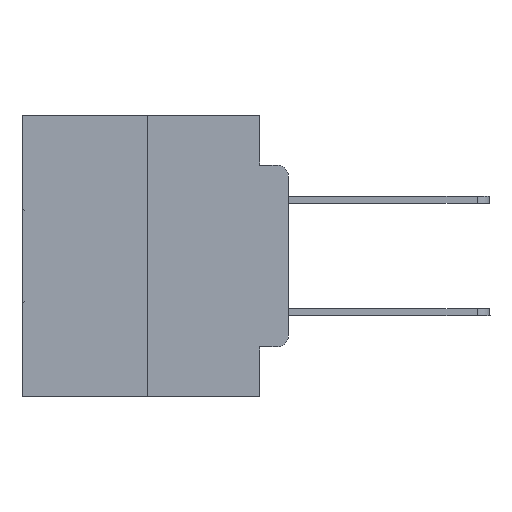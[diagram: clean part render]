
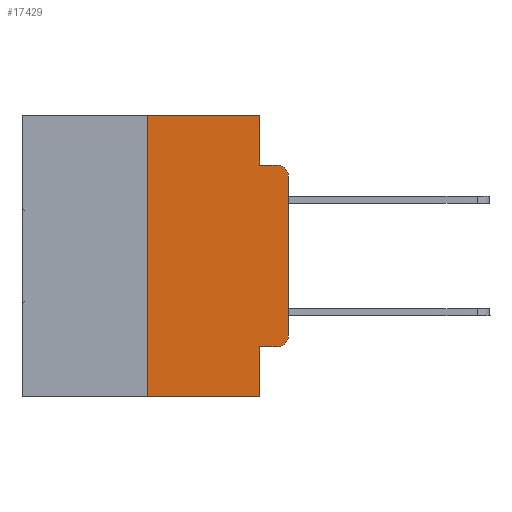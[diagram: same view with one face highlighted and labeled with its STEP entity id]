
A CAD part, left-side view. The second image highlights one B-rep face of the part: STEP entity #17429.
In plain terms, the highlighted planar face has unit normal (-1, 0, 0).
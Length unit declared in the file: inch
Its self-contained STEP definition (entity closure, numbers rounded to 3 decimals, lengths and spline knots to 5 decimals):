
#178 = CARTESIAN_POINT ( 'NONE',  ( 0., 0.473, 0. ) ) ;
#523 = CARTESIAN_POINT ( 'NONE',  ( 0., 0.473, 0. ) ) ;
#1475 = DIRECTION ( 'NONE',  ( 0., -1., 0. ) ) ;
#1770 = ORIENTED_EDGE ( 'NONE', *, *, #31047, .F. ) ;
#1960 = VERTEX_POINT ( 'NONE', #28649 ) ;
#2140 = LINE ( 'NONE', #178, #22435 ) ;
#2242 = DIRECTION ( 'NONE',  ( -1., 0., 0. ) ) ;
#3120 = DIRECTION ( 'NONE',  ( 0., -1., 0. ) ) ;
#4081 = LINE ( 'NONE', #28703, #7214 ) ;
#4144 = CARTESIAN_POINT ( 'NONE',  ( 0., 0.051, -0.0885 ) ) ;
#4491 = EDGE_CURVE ( 'NONE', #1960, #14045, #5254, .T. ) ;
#4605 = LINE ( 'NONE', #9718, #9971 ) ;
#5254 = LINE ( 'NONE', #29690, #6729 ) ;
#5444 = DIRECTION ( 'NONE',  ( 0., 0., -1. ) ) ;
#5607 = PLANE ( 'NONE',  #13604 ) ;
#5739 = CIRCLE ( 'NONE', #15173, 0.02 ) ;
#6519 = ORIENTED_EDGE ( 'NONE', *, *, #4491, .T. ) ;
#6729 = VECTOR ( 'NONE', #12666, 39.37008 ) ;
#7214 = VECTOR ( 'NONE', #1475, 39.37008 ) ;
#7254 = DIRECTION ( 'NONE',  ( 0., 0., 1. ) ) ;
#7322 = EDGE_CURVE ( 'NONE', #31018, #1960, #10816, .T. ) ;
#7426 = CARTESIAN_POINT ( 'NONE',  ( 0., 0.02, -0.3915 ) ) ;
#8475 = ORIENTED_EDGE ( 'NONE', *, *, #23157, .T. ) ;
#8695 = DIRECTION ( 'NONE',  ( 0., -1., 0. ) ) ;
#8791 = ORIENTED_EDGE ( 'NONE', *, *, #17737, .T. ) ;
#8928 = VERTEX_POINT ( 'NONE', #21375 ) ;
#9234 = AXIS2_PLACEMENT_3D ( 'NONE', #7426, #31680, #19246 ) ;
#9718 = CARTESIAN_POINT ( 'NONE',  ( 0., 0.25, 0. ) ) ;
#9971 = VECTOR ( 'NONE', #7254, 39.37008 ) ;
#10304 = ORIENTED_EDGE ( 'NONE', *, *, #13296, .F. ) ;
#10726 = EDGE_CURVE ( 'NONE', #16629, #25400, #2140, .T. ) ;
#10816 = CIRCLE ( 'NONE', #9234, 0.02 ) ;
#11049 = DIRECTION ( 'NONE',  ( 0., 0., -1. ) ) ;
#11190 = VERTEX_POINT ( 'NONE', #25070 ) ;
#11764 = DIRECTION ( 'NONE',  ( 0., 0., -1. ) ) ;
#12030 = CARTESIAN_POINT ( 'NONE',  ( 0., 0.02, -0.4115 ) ) ;
#12516 = ORIENTED_EDGE ( 'NONE', *, *, #7322, .T. ) ;
#12608 = CARTESIAN_POINT ( 'NONE',  ( 0., 0.02, -0.1085 ) ) ;
#12666 = DIRECTION ( 'NONE',  ( 0., 0., 1. ) ) ;
#13015 = DIRECTION ( 'NONE',  ( 1., 0., 0. ) ) ;
#13296 = EDGE_CURVE ( 'NONE', #18629, #11190, #21133, .T. ) ;
#13342 = FACE_OUTER_BOUND ( 'NONE', #28819, .T. ) ;
#13604 = AXIS2_PLACEMENT_3D ( 'NONE', #523, #13015, #5444 ) ;
#13749 = VECTOR ( 'NONE', #3120, 39.37008 ) ;
#13956 = VERTEX_POINT ( 'NONE', #18760 ) ;
#14045 = VERTEX_POINT ( 'NONE', #21718 ) ;
#14583 = EDGE_CURVE ( 'NONE', #13956, #11190, #4081, .T. ) ;
#15173 = AXIS2_PLACEMENT_3D ( 'NONE', #12608, #2242, #22620 ) ;
#16101 = LINE ( 'NONE', #30834, #13749 ) ;
#16122 = CARTESIAN_POINT ( 'NONE',  ( 0., 0.051, 0. ) ) ;
#16191 = EDGE_CURVE ( 'NONE', #22224, #8928, #21174, .T. ) ;
#16629 = VERTEX_POINT ( 'NONE', #23411 ) ;
#16900 = ORIENTED_EDGE ( 'NONE', *, *, #29596, .F. ) ;
#17429 = ADVANCED_FACE ( 'NONE', ( #13342 ), #5607, .F. ) ;
#17435 = DIRECTION ( 'NONE',  ( 0., -1., 0. ) ) ;
#17640 = VECTOR ( 'NONE', #11764, 39.37008 ) ;
#17737 = EDGE_CURVE ( 'NONE', #14045, #8928, #5739, .T. ) ;
#18629 = VERTEX_POINT ( 'NONE', #31448 ) ;
#18760 = CARTESIAN_POINT ( 'NONE',  ( 0., 0.25, -0.5 ) ) ;
#19246 = DIRECTION ( 'NONE',  ( 0., 0., -1. ) ) ;
#20957 = ORIENTED_EDGE ( 'NONE', *, *, #14583, .T. ) ;
#21133 = LINE ( 'NONE', #31573, #17640 ) ;
#21174 = LINE ( 'NONE', #31133, #25576 ) ;
#21375 = CARTESIAN_POINT ( 'NONE',  ( 0., 0.02, -0.0885 ) ) ;
#21718 = CARTESIAN_POINT ( 'NONE',  ( 0., 0., -0.1085 ) ) ;
#22224 = VERTEX_POINT ( 'NONE', #4144 ) ;
#22435 = VECTOR ( 'NONE', #17435, 39.37008 ) ;
#22620 = DIRECTION ( 'NONE',  ( 0., 0., -1. ) ) ;
#23157 = EDGE_CURVE ( 'NONE', #18629, #31018, #16101, .T. ) ;
#23411 = CARTESIAN_POINT ( 'NONE',  ( 0., 0.25, 0. ) ) ;
#23752 = ORIENTED_EDGE ( 'NONE', *, *, #16191, .F. ) ;
#25070 = CARTESIAN_POINT ( 'NONE',  ( 0., 0.051, -0.5 ) ) ;
#25400 = VERTEX_POINT ( 'NONE', #28153 ) ;
#25576 = VECTOR ( 'NONE', #8695, 39.37008 ) ;
#27500 = VECTOR ( 'NONE', #11049, 39.37008 ) ;
#27522 = ORIENTED_EDGE ( 'NONE', *, *, #10726, .F. ) ;
#28153 = CARTESIAN_POINT ( 'NONE',  ( 0., 0.051, 0. ) ) ;
#28649 = CARTESIAN_POINT ( 'NONE',  ( 0., 0., -0.3915 ) ) ;
#28703 = CARTESIAN_POINT ( 'NONE',  ( 0., 0.473, -0.5 ) ) ;
#28819 = EDGE_LOOP ( 'NONE', ( #6519, #8791, #23752, #16900, #27522, #1770, #20957, #10304, #8475, #12516 ) ) ;
#28866 = LINE ( 'NONE', #16122, #27500 ) ;
#29596 = EDGE_CURVE ( 'NONE', #25400, #22224, #28866, .T. ) ;
#29690 = CARTESIAN_POINT ( 'NONE',  ( 0., 0., 0. ) ) ;
#30834 = CARTESIAN_POINT ( 'NONE',  ( 0., 0.051, -0.4115 ) ) ;
#31018 = VERTEX_POINT ( 'NONE', #12030 ) ;
#31047 = EDGE_CURVE ( 'NONE', #13956, #16629, #4605, .T. ) ;
#31133 = CARTESIAN_POINT ( 'NONE',  ( 0., 0.051, -0.0885 ) ) ;
#31448 = CARTESIAN_POINT ( 'NONE',  ( 0., 0.051, -0.4115 ) ) ;
#31573 = CARTESIAN_POINT ( 'NONE',  ( 0., 0.051, 0. ) ) ;
#31680 = DIRECTION ( 'NONE',  ( -1., 0., 0. ) ) ;
